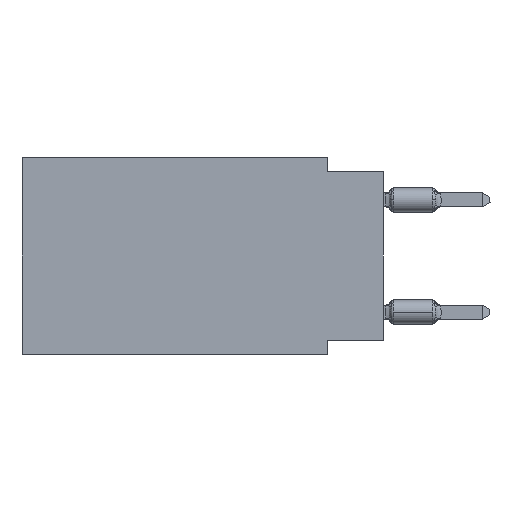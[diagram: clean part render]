
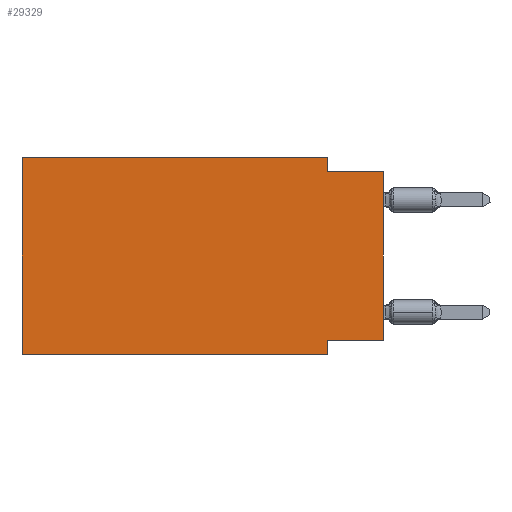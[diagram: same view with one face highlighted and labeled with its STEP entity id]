
A CAD part, left-side view. The second image highlights one B-rep face of the part: STEP entity #29329.
In plain terms, the highlighted planar face has unit normal (-1, 0, 0).
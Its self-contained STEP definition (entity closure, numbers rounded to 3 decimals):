
#126 = CARTESIAN_POINT ( 'NONE',  ( 0., 0., -0.635 ) ) ;
#628 = CARTESIAN_POINT ( 'NONE',  ( 0., 0., -0.635 ) ) ;
#894 = CARTESIAN_POINT ( 'NONE',  ( 0., 16.383, 0. ) ) ;
#1940 = VECTOR ( 'NONE', #11580, 1000. ) ;
#1976 = VECTOR ( 'NONE', #24035, 1000. ) ;
#2216 = CARTESIAN_POINT ( 'NONE',  ( 0., 2.54, -8.89 ) ) ;
#3305 = VERTEX_POINT ( 'NONE', #894 ) ;
#3569 = ORIENTED_EDGE ( 'NONE', *, *, #17873, .F. ) ;
#4321 = DIRECTION ( 'NONE',  ( 1., 0., 0. ) ) ;
#4662 = CARTESIAN_POINT ( 'NONE',  ( 0., 16.383, 0. ) ) ;
#4751 = VERTEX_POINT ( 'NONE', #2216 ) ;
#6083 = CARTESIAN_POINT ( 'NONE',  ( 0., 16.383, 0. ) ) ;
#6466 = CARTESIAN_POINT ( 'NONE',  ( 0., 0., 0. ) ) ;
#7180 = CARTESIAN_POINT ( 'NONE',  ( 0., 0., -8.255 ) ) ;
#8055 = CARTESIAN_POINT ( 'NONE',  ( 0., 16.383, 0. ) ) ;
#8117 = VERTEX_POINT ( 'NONE', #126 ) ;
#8530 = CARTESIAN_POINT ( 'NONE',  ( 0., 0., -8.255 ) ) ;
#9322 = VECTOR ( 'NONE', #10879, 1000. ) ;
#9524 = LINE ( 'NONE', #17182, #28434 ) ;
#9653 = EDGE_CURVE ( 'NONE', #15440, #4751, #31583, .T. ) ;
#10376 = LINE ( 'NONE', #8055, #31233 ) ;
#10556 = CARTESIAN_POINT ( 'NONE',  ( 0., 2.54, -8.89 ) ) ;
#10879 = DIRECTION ( 'NONE',  ( 0., 0., -1. ) ) ;
#10902 = EDGE_CURVE ( 'NONE', #19725, #17693, #9524, .T. ) ;
#11580 = DIRECTION ( 'NONE',  ( 0., 0., 1. ) ) ;
#11909 = LINE ( 'NONE', #6466, #1940 ) ;
#12115 = ORIENTED_EDGE ( 'NONE', *, *, #10902, .F. ) ;
#12397 = CARTESIAN_POINT ( 'NONE',  ( 0., 2.54, -0.635 ) ) ;
#13356 = VERTEX_POINT ( 'NONE', #7180 ) ;
#13619 = CARTESIAN_POINT ( 'NONE',  ( 0., 16.383, -8.89 ) ) ;
#15086 = EDGE_CURVE ( 'NONE', #15440, #3305, #23382, .T. ) ;
#15161 = ORIENTED_EDGE ( 'NONE', *, *, #24233, .T. ) ;
#15440 = VERTEX_POINT ( 'NONE', #29600 ) ;
#15800 = EDGE_LOOP ( 'NONE', ( #15161, #24776, #12115, #16382, #26915, #31495, #3569, #31088 ) ) ;
#16382 = ORIENTED_EDGE ( 'NONE', *, *, #26208, .F. ) ;
#17182 = CARTESIAN_POINT ( 'NONE',  ( 0., 2.54, 0. ) ) ;
#17693 = VERTEX_POINT ( 'NONE', #12397 ) ;
#17873 = EDGE_CURVE ( 'NONE', #23941, #4751, #18628, .T. ) ;
#18119 = DIRECTION ( 'NONE',  ( 0., -1., 0. ) ) ;
#18280 = LINE ( 'NONE', #628, #24413 ) ;
#18628 = LINE ( 'NONE', #10556, #9322 ) ;
#18729 = CARTESIAN_POINT ( 'NONE',  ( 0., 2.54, 0. ) ) ;
#19725 = VERTEX_POINT ( 'NONE', #18729 ) ;
#21214 = LINE ( 'NONE', #8530, #24657 ) ;
#21634 = FACE_OUTER_BOUND ( 'NONE', #15800, .T. ) ;
#23286 = EDGE_CURVE ( 'NONE', #13356, #23941, #21214, .T. ) ;
#23382 = LINE ( 'NONE', #6083, #1976 ) ;
#23941 = VERTEX_POINT ( 'NONE', #30221 ) ;
#24035 = DIRECTION ( 'NONE',  ( 0., 0., 1. ) ) ;
#24233 = EDGE_CURVE ( 'NONE', #13356, #8117, #11909, .T. ) ;
#24413 = VECTOR ( 'NONE', #18119, 1000. ) ;
#24657 = VECTOR ( 'NONE', #30939, 1000. ) ;
#24776 = ORIENTED_EDGE ( 'NONE', *, *, #26246, .F. ) ;
#26208 = EDGE_CURVE ( 'NONE', #3305, #19725, #10376, .T. ) ;
#26246 = EDGE_CURVE ( 'NONE', #17693, #8117, #18280, .T. ) ;
#26651 = AXIS2_PLACEMENT_3D ( 'NONE', #4662, #4321, #29700 ) ;
#26801 = VECTOR ( 'NONE', #28942, 1000. ) ;
#26915 = ORIENTED_EDGE ( 'NONE', *, *, #15086, .F. ) ;
#27222 = DIRECTION ( 'NONE',  ( 0., 0., -1. ) ) ;
#28434 = VECTOR ( 'NONE', #27222, 1000. ) ;
#28942 = DIRECTION ( 'NONE',  ( 0., -1., 0. ) ) ;
#29329 = ADVANCED_FACE ( 'NONE', ( #21634 ), #29532, .F. ) ;
#29532 = PLANE ( 'NONE',  #26651 ) ;
#29600 = CARTESIAN_POINT ( 'NONE',  ( 0., 16.383, -8.89 ) ) ;
#29700 = DIRECTION ( 'NONE',  ( 0., 0., -1. ) ) ;
#30221 = CARTESIAN_POINT ( 'NONE',  ( 0., 2.54, -8.255 ) ) ;
#30939 = DIRECTION ( 'NONE',  ( 0., 1., 0. ) ) ;
#30951 = DIRECTION ( 'NONE',  ( 0., -1., 0. ) ) ;
#31088 = ORIENTED_EDGE ( 'NONE', *, *, #23286, .F. ) ;
#31233 = VECTOR ( 'NONE', #30951, 1000. ) ;
#31495 = ORIENTED_EDGE ( 'NONE', *, *, #9653, .T. ) ;
#31583 = LINE ( 'NONE', #13619, #26801 ) ;
